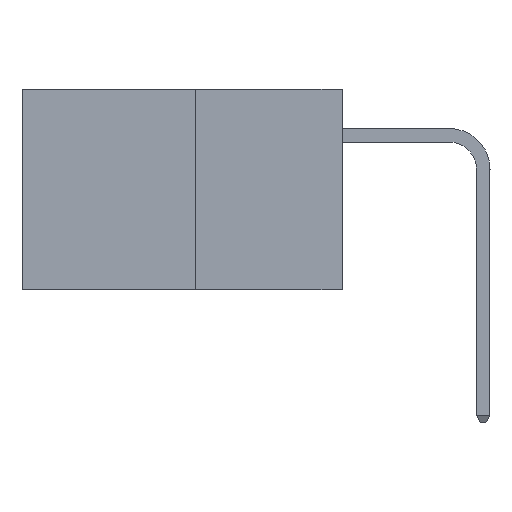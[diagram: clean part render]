
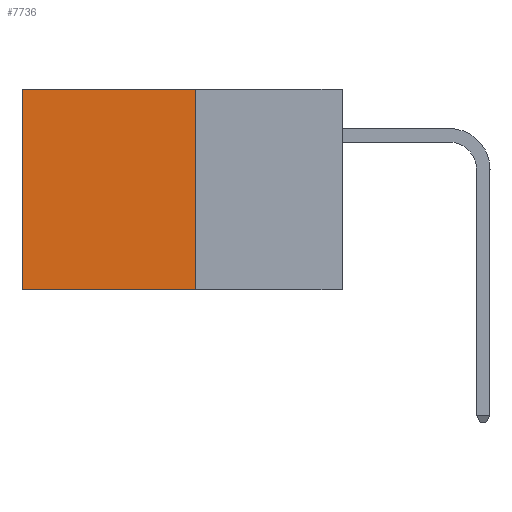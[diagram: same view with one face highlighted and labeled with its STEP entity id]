
A CAD part, left-side view. The second image highlights one B-rep face of the part: STEP entity #7736.
In plain terms, the highlighted planar face has unit normal (-1, 0, 0).
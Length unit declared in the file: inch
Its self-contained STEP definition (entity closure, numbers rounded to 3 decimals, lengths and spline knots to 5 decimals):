
#11 = DIRECTION ( 'NONE',  ( 0., 0., -1. ) ) ;
#941 = CARTESIAN_POINT ( 'NONE',  ( 0.277, 0.27, -0.37 ) ) ;
#1125 = CARTESIAN_POINT ( 'NONE',  ( 0.277, 0.59, -0.37 ) ) ;
#1253 = LINE ( 'NONE', #17990, #27560 ) ;
#1654 = AXIS2_PLACEMENT_3D ( 'NONE', #941, #26486, #11315 ) ;
#2513 = CARTESIAN_POINT ( 'NONE',  ( 0.277, 0.27, 0. ) ) ;
#5911 = EDGE_CURVE ( 'NONE', #19783, #18695, #10731, .T. ) ;
#6450 = DIRECTION ( 'NONE',  ( 0., 1., 0. ) ) ;
#7736 = ADVANCED_FACE ( 'NONE', ( #31552 ), #23993, .F. ) ;
#8476 = EDGE_LOOP ( 'NONE', ( #28135, #18739, #15443, #23568 ) ) ;
#8899 = VECTOR ( 'NONE', #12896, 39.37008 ) ;
#9124 = VECTOR ( 'NONE', #21895, 39.37008 ) ;
#9607 = EDGE_CURVE ( 'NONE', #26604, #19783, #10516, .T. ) ;
#10516 = LINE ( 'NONE', #2513, #8899 ) ;
#10731 = LINE ( 'NONE', #1125, #9124 ) ;
#11315 = DIRECTION ( 'NONE',  ( 0., 0., -1. ) ) ;
#12896 = DIRECTION ( 'NONE',  ( 0., 1., 0. ) ) ;
#13936 = VECTOR ( 'NONE', #6450, 39.37008 ) ;
#14711 = LINE ( 'NONE', #31705, #13936 ) ;
#15041 = CARTESIAN_POINT ( 'NONE',  ( 0.277, 0.27, -0.37 ) ) ;
#15443 = ORIENTED_EDGE ( 'NONE', *, *, #27434, .F. ) ;
#16675 = CARTESIAN_POINT ( 'NONE',  ( 0.277, 0.27, 0. ) ) ;
#17990 = CARTESIAN_POINT ( 'NONE',  ( 0.277, 0.27, -0.37 ) ) ;
#18695 = VERTEX_POINT ( 'NONE', #27404 ) ;
#18739 = ORIENTED_EDGE ( 'NONE', *, *, #24565, .F. ) ;
#19154 = CARTESIAN_POINT ( 'NONE',  ( 0.277, 0.59, 0. ) ) ;
#19783 = VERTEX_POINT ( 'NONE', #19154 ) ;
#21273 = VERTEX_POINT ( 'NONE', #15041 ) ;
#21895 = DIRECTION ( 'NONE',  ( 0., 0., -1. ) ) ;
#23568 = ORIENTED_EDGE ( 'NONE', *, *, #9607, .T. ) ;
#23993 = PLANE ( 'NONE',  #1654 ) ;
#24565 = EDGE_CURVE ( 'NONE', #21273, #18695, #14711, .T. ) ;
#26486 = DIRECTION ( 'NONE',  ( 1., 0., 0. ) ) ;
#26604 = VERTEX_POINT ( 'NONE', #16675 ) ;
#27404 = CARTESIAN_POINT ( 'NONE',  ( 0.277, 0.59, -0.37 ) ) ;
#27434 = EDGE_CURVE ( 'NONE', #26604, #21273, #1253, .T. ) ;
#27560 = VECTOR ( 'NONE', #11, 39.37008 ) ;
#28135 = ORIENTED_EDGE ( 'NONE', *, *, #5911, .T. ) ;
#31552 = FACE_OUTER_BOUND ( 'NONE', #8476, .T. ) ;
#31705 = CARTESIAN_POINT ( 'NONE',  ( 0.277, 0.27, -0.37 ) ) ;
